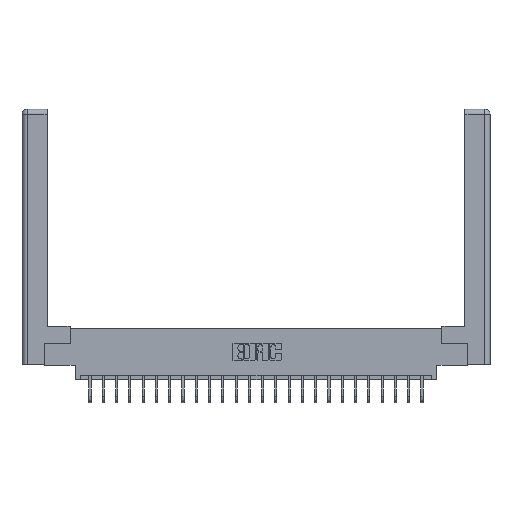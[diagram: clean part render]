
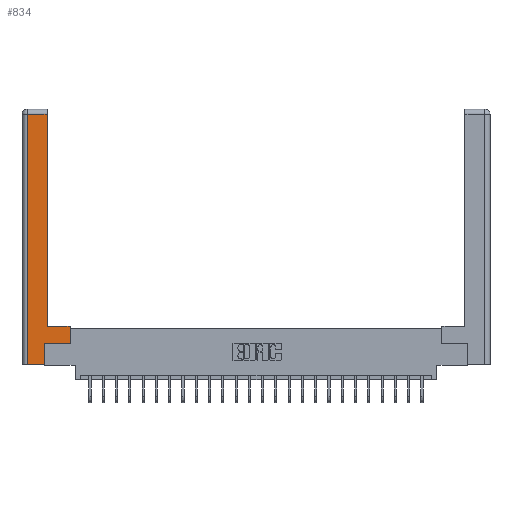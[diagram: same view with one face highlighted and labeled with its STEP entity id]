
A CAD part, top view. The second image highlights one B-rep face of the part: STEP entity #834.
In plain terms, the highlighted planar face has unit normal (0, 0, 1).
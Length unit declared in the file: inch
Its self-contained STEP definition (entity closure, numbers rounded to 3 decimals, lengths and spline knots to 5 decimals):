
#338 = ORIENTED_EDGE ( 'NONE', *, *, #5161, .T. ) ;
#834 = ADVANCED_FACE ( 'NONE', ( #22090 ), #19843, .F. ) ;
#1012 = DIRECTION ( 'NONE',  ( -1., 0., 0. ) ) ;
#1221 = LINE ( 'NONE', #14160, #22948 ) ;
#1305 = CARTESIAN_POINT ( 'NONE',  ( 0.565, 0.45, 0. ) ) ;
#1415 = VECTOR ( 'NONE', #11258, 39.37008 ) ;
#1463 = DIRECTION ( 'NONE',  ( -1., 0., 0. ) ) ;
#1464 = CARTESIAN_POINT ( 'NONE',  ( 0.0615, 0., 0. ) ) ;
#1816 = ORIENTED_EDGE ( 'NONE', *, *, #14815, .T. ) ;
#2079 = EDGE_CURVE ( 'NONE', #6397, #18290, #19730, .T. ) ;
#2995 = CARTESIAN_POINT ( 'NONE',  ( 0.565, 0.245, 0. ) ) ;
#3190 = CARTESIAN_POINT ( 'NONE',  ( 0.265, 0., 0. ) ) ;
#3288 = CARTESIAN_POINT ( 'NONE',  ( 0.295, 2.94, 0. ) ) ;
#3547 = EDGE_CURVE ( 'NONE', #18290, #20243, #4142, .T. ) ;
#3551 = DIRECTION ( 'NONE',  ( 0., 1., 0. ) ) ;
#4142 = LINE ( 'NONE', #13197, #20001 ) ;
#4839 = DIRECTION ( 'NONE',  ( 1., 0., 0. ) ) ;
#5161 = EDGE_CURVE ( 'NONE', #20641, #8663, #26333, .T. ) ;
#5405 = CARTESIAN_POINT ( 'NONE',  ( 0.0615, 0., 0. ) ) ;
#5494 = CARTESIAN_POINT ( 'NONE',  ( 0.265, 0.245, 0. ) ) ;
#5644 = EDGE_CURVE ( 'NONE', #17689, #20641, #24065, .T. ) ;
#6397 = VERTEX_POINT ( 'NONE', #22458 ) ;
#7285 = DIRECTION ( 'NONE',  ( 0., 0., -1. ) ) ;
#7493 = DIRECTION ( 'NONE',  ( 0., -1., 0. ) ) ;
#7571 = VECTOR ( 'NONE', #1463, 39.37008 ) ;
#7572 = ORIENTED_EDGE ( 'NONE', *, *, #3547, .T. ) ;
#8663 = VERTEX_POINT ( 'NONE', #3288 ) ;
#8700 = EDGE_CURVE ( 'NONE', #8663, #25244, #1221, .T. ) ;
#9515 = VECTOR ( 'NONE', #15926, 39.37008 ) ;
#10459 = EDGE_CURVE ( 'NONE', #21459, #6397, #10720, .T. ) ;
#10720 = LINE ( 'NONE', #3190, #24295 ) ;
#11258 = DIRECTION ( 'NONE',  ( 0., 1., 0. ) ) ;
#11651 = CARTESIAN_POINT ( 'NONE',  ( 0., 0., 0. ) ) ;
#12827 = LINE ( 'NONE', #5405, #25711 ) ;
#13197 = CARTESIAN_POINT ( 'NONE',  ( 0.565, 0.245, 0. ) ) ;
#13704 = CARTESIAN_POINT ( 'NONE',  ( 0.295, 0.45, 0. ) ) ;
#14158 = CARTESIAN_POINT ( 'NONE',  ( 0.265, 0.245, 0. ) ) ;
#14160 = CARTESIAN_POINT ( 'NONE',  ( 0.0615, 2.94, 0. ) ) ;
#14408 = CARTESIAN_POINT ( 'NONE',  ( 0.295, 0.45, 0. ) ) ;
#14815 = EDGE_CURVE ( 'NONE', #20243, #17689, #17597, .T. ) ;
#14827 = ORIENTED_EDGE ( 'NONE', *, *, #5644, .T. ) ;
#15762 = ORIENTED_EDGE ( 'NONE', *, *, #2079, .T. ) ;
#15926 = DIRECTION ( 'NONE',  ( 0., 1., 0. ) ) ;
#17064 = AXIS2_PLACEMENT_3D ( 'NONE', #11651, #7285, #1012 ) ;
#17587 = CARTESIAN_POINT ( 'NONE',  ( 0.0615, 2.94, 0. ) ) ;
#17597 = LINE ( 'NONE', #26494, #9515 ) ;
#17689 = VERTEX_POINT ( 'NONE', #1305 ) ;
#18261 = EDGE_CURVE ( 'NONE', #25244, #21459, #12827, .T. ) ;
#18290 = VERTEX_POINT ( 'NONE', #5494 ) ;
#19730 = LINE ( 'NONE', #14158, #20390 ) ;
#19843 = PLANE ( 'NONE',  #17064 ) ;
#20001 = VECTOR ( 'NONE', #4839, 39.37008 ) ;
#20243 = VERTEX_POINT ( 'NONE', #2995 ) ;
#20390 = VECTOR ( 'NONE', #3551, 39.37008 ) ;
#20641 = VERTEX_POINT ( 'NONE', #14408 ) ;
#21456 = CARTESIAN_POINT ( 'NONE',  ( 0.295, 3., 0. ) ) ;
#21459 = VERTEX_POINT ( 'NONE', #1464 ) ;
#22090 = FACE_OUTER_BOUND ( 'NONE', #25021, .T. ) ;
#22116 = DIRECTION ( 'NONE',  ( 1., 0., 0. ) ) ;
#22458 = CARTESIAN_POINT ( 'NONE',  ( 0.265, 0., 0. ) ) ;
#22948 = VECTOR ( 'NONE', #26359, 39.37008 ) ;
#24065 = LINE ( 'NONE', #13704, #7571 ) ;
#24295 = VECTOR ( 'NONE', #22116, 39.37008 ) ;
#24769 = ORIENTED_EDGE ( 'NONE', *, *, #8700, .T. ) ;
#24844 = ORIENTED_EDGE ( 'NONE', *, *, #10459, .T. ) ;
#25021 = EDGE_LOOP ( 'NONE', ( #338, #24769, #25795, #24844, #15762, #7572, #1816, #14827 ) ) ;
#25244 = VERTEX_POINT ( 'NONE', #17587 ) ;
#25711 = VECTOR ( 'NONE', #7493, 39.37008 ) ;
#25795 = ORIENTED_EDGE ( 'NONE', *, *, #18261, .T. ) ;
#26333 = LINE ( 'NONE', #21456, #1415 ) ;
#26359 = DIRECTION ( 'NONE',  ( -1., 0., 0. ) ) ;
#26494 = CARTESIAN_POINT ( 'NONE',  ( 0.565, 0.45, 0. ) ) ;
